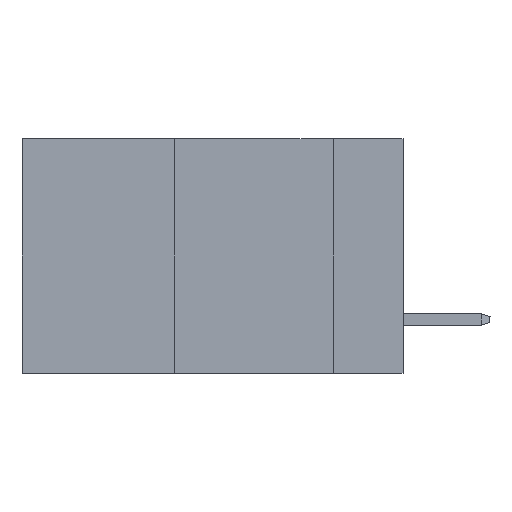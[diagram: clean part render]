
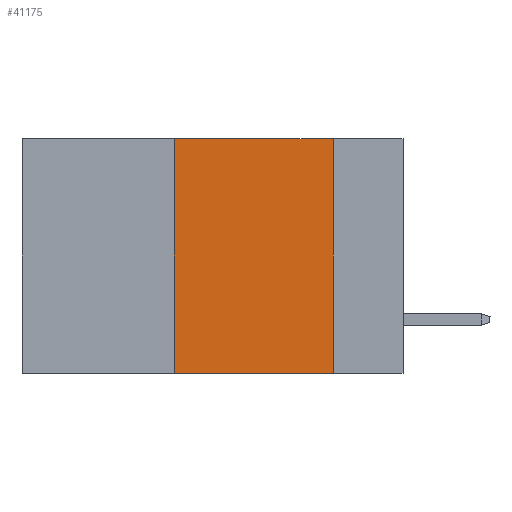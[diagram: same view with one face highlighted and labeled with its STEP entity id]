
A CAD part, left-side view. The second image highlights one B-rep face of the part: STEP entity #41175.
In plain terms, the highlighted planar face has unit normal (-1, 0, 0).
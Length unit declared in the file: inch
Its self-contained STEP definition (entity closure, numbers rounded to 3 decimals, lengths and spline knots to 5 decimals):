
#202 = VECTOR ( 'NONE', #9956, 39.37008 ) ;
#1490 = LINE ( 'NONE', #30977, #23381 ) ;
#1887 = DIRECTION ( 'NONE',  ( 0., -1., 0. ) ) ;
#4688 = DIRECTION ( 'NONE',  ( 0., -1., 0. ) ) ;
#5268 = CARTESIAN_POINT ( 'NONE',  ( 0., 0.36, 0. ) ) ;
#9226 = VERTEX_POINT ( 'NONE', #5268 ) ;
#9956 = DIRECTION ( 'NONE',  ( 0., 0., -1. ) ) ;
#10395 = DIRECTION ( 'NONE',  ( 0., 0., 1. ) ) ;
#12673 = DIRECTION ( 'NONE',  ( 1., 0., 0. ) ) ;
#13152 = CARTESIAN_POINT ( 'NONE',  ( 0., 0.11, -0.37 ) ) ;
#13336 = VERTEX_POINT ( 'NONE', #38946 ) ;
#13615 = LINE ( 'NONE', #31807, #202 ) ;
#14678 = ORIENTED_EDGE ( 'NONE', *, *, #38884, .F. ) ;
#14705 = VERTEX_POINT ( 'NONE', #13152 ) ;
#15806 = ORIENTED_EDGE ( 'NONE', *, *, #41225, .T. ) ;
#20188 = ORIENTED_EDGE ( 'NONE', *, *, #39043, .F. ) ;
#21386 = ORIENTED_EDGE ( 'NONE', *, *, #30059, .F. ) ;
#23381 = VECTOR ( 'NONE', #4688, 39.37008 ) ;
#24226 = FACE_OUTER_BOUND ( 'NONE', #42522, .T. ) ;
#25748 = VECTOR ( 'NONE', #10395, 39.37008 ) ;
#26564 = AXIS2_PLACEMENT_3D ( 'NONE', #32330, #12673, #46557 ) ;
#27906 = LINE ( 'NONE', #42872, #30491 ) ;
#30059 = EDGE_CURVE ( 'NONE', #36710, #14705, #13615, .T. ) ;
#30491 = VECTOR ( 'NONE', #1887, 39.37008 ) ;
#30977 = CARTESIAN_POINT ( 'NONE',  ( 0., 0.6, 0. ) ) ;
#31807 = CARTESIAN_POINT ( 'NONE',  ( 0., 0.11, 0. ) ) ;
#32330 = CARTESIAN_POINT ( 'NONE',  ( 0., 0.6, 0. ) ) ;
#33677 = LINE ( 'NONE', #48411, #25748 ) ;
#35766 = PLANE ( 'NONE',  #26564 ) ;
#36710 = VERTEX_POINT ( 'NONE', #37586 ) ;
#37586 = CARTESIAN_POINT ( 'NONE',  ( 0., 0.11, 0. ) ) ;
#38884 = EDGE_CURVE ( 'NONE', #13336, #9226, #33677, .T. ) ;
#38946 = CARTESIAN_POINT ( 'NONE',  ( 0., 0.36, -0.37 ) ) ;
#39043 = EDGE_CURVE ( 'NONE', #9226, #36710, #1490, .T. ) ;
#41175 = ADVANCED_FACE ( 'NONE', ( #24226 ), #35766, .F. ) ;
#41225 = EDGE_CURVE ( 'NONE', #13336, #14705, #27906, .T. ) ;
#42522 = EDGE_LOOP ( 'NONE', ( #21386, #20188, #14678, #15806 ) ) ;
#42872 = CARTESIAN_POINT ( 'NONE',  ( 0., 0.6, -0.37 ) ) ;
#46557 = DIRECTION ( 'NONE',  ( 0., 0., -1. ) ) ;
#48411 = CARTESIAN_POINT ( 'NONE',  ( 0., 0.36, 0. ) ) ;
